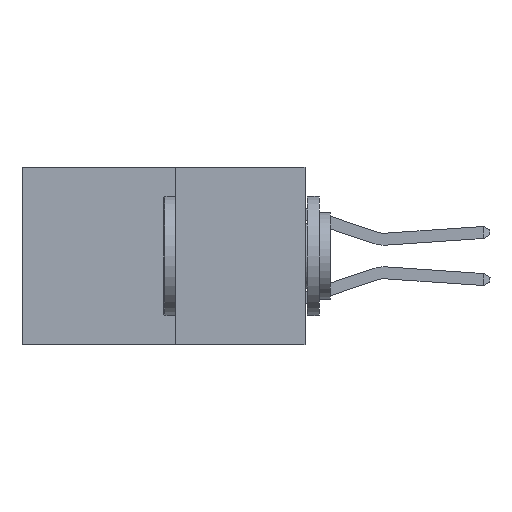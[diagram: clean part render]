
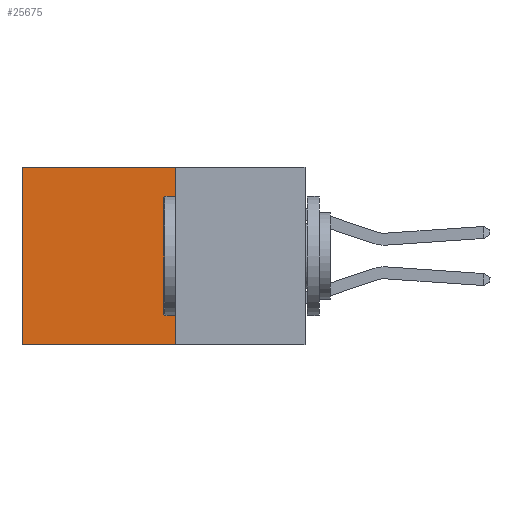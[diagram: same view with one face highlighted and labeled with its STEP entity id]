
A CAD part, left-side view. The second image highlights one B-rep face of the part: STEP entity #25675.
In plain terms, the highlighted planar face has unit normal (-1, 0, 0).
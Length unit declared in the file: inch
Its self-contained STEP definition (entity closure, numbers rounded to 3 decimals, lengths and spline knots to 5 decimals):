
#1075 = LINE ( 'NONE', #4866, #20191 ) ;
#1869 = EDGE_CURVE ( 'NONE', #11779, #22917, #1075, .T. ) ;
#2173 = DIRECTION ( 'NONE',  ( 0., 0., -1. ) ) ;
#2802 = CARTESIAN_POINT ( 'NONE',  ( 0.277, 0.59, -0.37 ) ) ;
#3992 = EDGE_CURVE ( 'NONE', #22917, #12195, #18881, .T. ) ;
#4866 = CARTESIAN_POINT ( 'NONE',  ( 0.277, 0.27, 0. ) ) ;
#5069 = VECTOR ( 'NONE', #26703, 39.37008 ) ;
#5314 = ORIENTED_EDGE ( 'NONE', *, *, #3992, .T. ) ;
#7059 = CARTESIAN_POINT ( 'NONE',  ( 0.277, 0.27, -0.37 ) ) ;
#8107 = VECTOR ( 'NONE', #14189, 39.37008 ) ;
#9149 = CARTESIAN_POINT ( 'NONE',  ( 0.277, 0.27, -0.37 ) ) ;
#10049 = EDGE_LOOP ( 'NONE', ( #5314, #21807, #28556, #18796 ) ) ;
#10891 = LINE ( 'NONE', #16605, #5069 ) ;
#11079 = FACE_OUTER_BOUND ( 'NONE', #10049, .T. ) ;
#11779 = VERTEX_POINT ( 'NONE', #28822 ) ;
#12195 = VERTEX_POINT ( 'NONE', #2802 ) ;
#12920 = CARTESIAN_POINT ( 'NONE',  ( 0.277, 0.27, -0.37 ) ) ;
#14189 = DIRECTION ( 'NONE',  ( 0., 1., 0. ) ) ;
#14607 = PLANE ( 'NONE',  #23704 ) ;
#16318 = EDGE_CURVE ( 'NONE', #11779, #21250, #10891, .T. ) ;
#16605 = CARTESIAN_POINT ( 'NONE',  ( 0.277, 0.27, -0.37 ) ) ;
#17097 = DIRECTION ( 'NONE',  ( 1., 0., 0. ) ) ;
#18796 = ORIENTED_EDGE ( 'NONE', *, *, #1869, .T. ) ;
#18881 = LINE ( 'NONE', #31951, #31422 ) ;
#20191 = VECTOR ( 'NONE', #22298, 39.37008 ) ;
#21250 = VERTEX_POINT ( 'NONE', #12920 ) ;
#21402 = LINE ( 'NONE', #9149, #8107 ) ;
#21807 = ORIENTED_EDGE ( 'NONE', *, *, #23482, .F. ) ;
#22298 = DIRECTION ( 'NONE',  ( 0., 1., 0. ) ) ;
#22917 = VERTEX_POINT ( 'NONE', #24087 ) ;
#23482 = EDGE_CURVE ( 'NONE', #21250, #12195, #21402, .T. ) ;
#23704 = AXIS2_PLACEMENT_3D ( 'NONE', #7059, #17097, #2173 ) ;
#24087 = CARTESIAN_POINT ( 'NONE',  ( 0.277, 0.59, 0. ) ) ;
#25675 = ADVANCED_FACE ( 'NONE', ( #11079 ), #14607, .F. ) ;
#26703 = DIRECTION ( 'NONE',  ( 0., 0., -1. ) ) ;
#28556 = ORIENTED_EDGE ( 'NONE', *, *, #16318, .F. ) ;
#28822 = CARTESIAN_POINT ( 'NONE',  ( 0.277, 0.27, 0. ) ) ;
#31283 = DIRECTION ( 'NONE',  ( 0., 0., -1. ) ) ;
#31422 = VECTOR ( 'NONE', #31283, 39.37008 ) ;
#31951 = CARTESIAN_POINT ( 'NONE',  ( 0.277, 0.59, -0.37 ) ) ;
